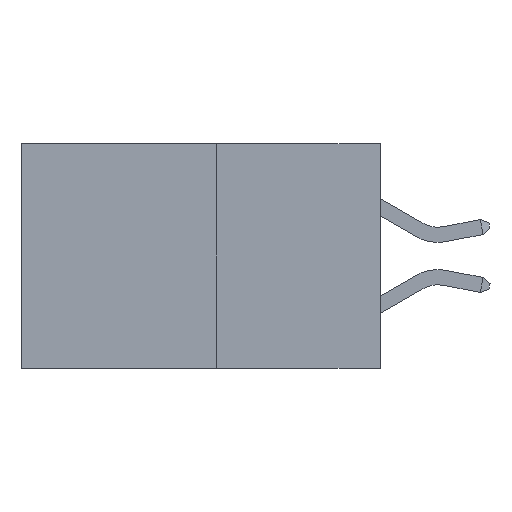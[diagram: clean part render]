
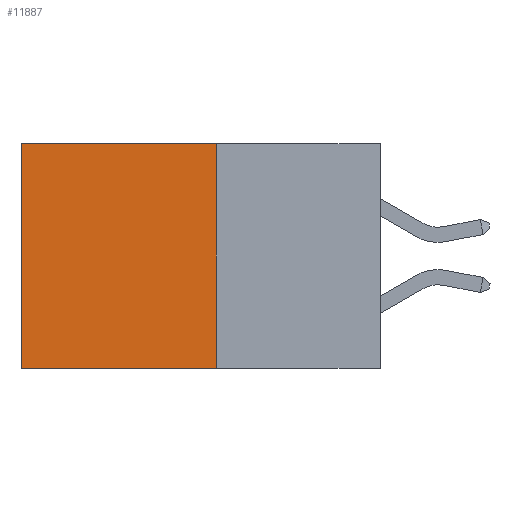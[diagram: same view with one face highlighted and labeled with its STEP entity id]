
A CAD part, left-side view. The second image highlights one B-rep face of the part: STEP entity #11887.
In plain terms, the highlighted planar face has unit normal (-1, 0, 0).
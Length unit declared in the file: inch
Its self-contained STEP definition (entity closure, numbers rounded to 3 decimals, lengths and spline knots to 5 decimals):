
#3 = VECTOR ( 'NONE', #8847, 39.37008 ) ;
#102 = CARTESIAN_POINT ( 'NONE',  ( 0.277, 0.27, -0.37 ) ) ;
#233 = AXIS2_PLACEMENT_3D ( 'NONE', #102, #1100, #8310 ) ;
#286 = CARTESIAN_POINT ( 'NONE',  ( 0.277, 0.27, 0. ) ) ;
#683 = EDGE_CURVE ( 'NONE', #1910, #2607, #6157, .T. ) ;
#840 = CARTESIAN_POINT ( 'NONE',  ( 0.277, 0.59, 0. ) ) ;
#956 = ORIENTED_EDGE ( 'NONE', *, *, #11131, .T. ) ;
#1100 = DIRECTION ( 'NONE',  ( 1., 0., 0. ) ) ;
#1910 = VERTEX_POINT ( 'NONE', #2132 ) ;
#2132 = CARTESIAN_POINT ( 'NONE',  ( 0.277, 0.27, 0. ) ) ;
#2205 = CARTESIAN_POINT ( 'NONE',  ( 0.277, 0.59, -0.37 ) ) ;
#2219 = VECTOR ( 'NONE', #8513, 39.37008 ) ;
#2493 = EDGE_CURVE ( 'NONE', #2607, #12036, #2685, .T. ) ;
#2607 = VERTEX_POINT ( 'NONE', #5072 ) ;
#2685 = LINE ( 'NONE', #2882, #3 ) ;
#2882 = CARTESIAN_POINT ( 'NONE',  ( 0.277, 0.27, -0.37 ) ) ;
#4978 = EDGE_CURVE ( 'NONE', #11652, #12036, #8791, .T. ) ;
#5072 = CARTESIAN_POINT ( 'NONE',  ( 0.277, 0.27, -0.37 ) ) ;
#6157 = LINE ( 'NONE', #11891, #11172 ) ;
#6570 = ORIENTED_EDGE ( 'NONE', *, *, #4978, .T. ) ;
#7703 = FACE_OUTER_BOUND ( 'NONE', #12222, .T. ) ;
#8310 = DIRECTION ( 'NONE',  ( 0., 0., -1. ) ) ;
#8461 = VECTOR ( 'NONE', #9582, 39.37008 ) ;
#8513 = DIRECTION ( 'NONE',  ( 0., 1., 0. ) ) ;
#8791 = LINE ( 'NONE', #9901, #8461 ) ;
#8847 = DIRECTION ( 'NONE',  ( 0., 1., 0. ) ) ;
#9316 = ORIENTED_EDGE ( 'NONE', *, *, #2493, .F. ) ;
#9582 = DIRECTION ( 'NONE',  ( 0., 0., -1. ) ) ;
#9595 = DIRECTION ( 'NONE',  ( 0., 0., -1. ) ) ;
#9901 = CARTESIAN_POINT ( 'NONE',  ( 0.277, 0.59, -0.37 ) ) ;
#10384 = LINE ( 'NONE', #286, #2219 ) ;
#10816 = ORIENTED_EDGE ( 'NONE', *, *, #683, .F. ) ;
#11131 = EDGE_CURVE ( 'NONE', #1910, #11652, #10384, .T. ) ;
#11172 = VECTOR ( 'NONE', #9595, 39.37008 ) ;
#11652 = VERTEX_POINT ( 'NONE', #840 ) ;
#11887 = ADVANCED_FACE ( 'NONE', ( #7703 ), #12086, .F. ) ;
#11891 = CARTESIAN_POINT ( 'NONE',  ( 0.277, 0.27, -0.37 ) ) ;
#12036 = VERTEX_POINT ( 'NONE', #2205 ) ;
#12086 = PLANE ( 'NONE',  #233 ) ;
#12222 = EDGE_LOOP ( 'NONE', ( #6570, #9316, #10816, #956 ) ) ;
